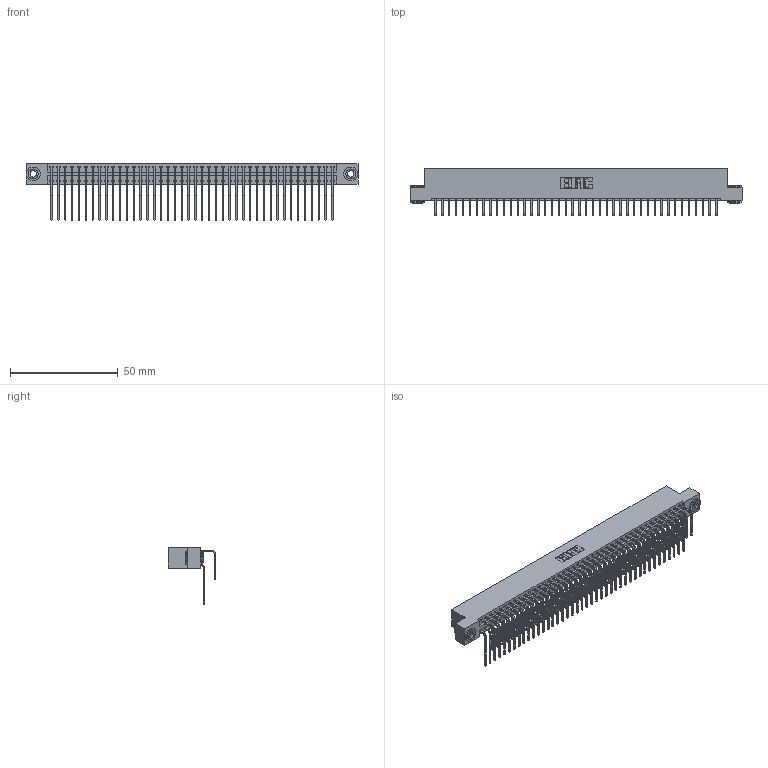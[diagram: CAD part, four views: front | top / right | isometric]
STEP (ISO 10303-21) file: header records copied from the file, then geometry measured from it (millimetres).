
FILE_DESCRIPTION (( 'STEP AP203' ), '1' );
FILE_NAME ('346-084-558-203.STEP', '2022-05-25T20:49:17', ( '' ), ( '' ), 'SwSTEP 2.0', 'SolidWorks 2020', '' );
FILE_SCHEMA (( 'CONFIG_CONTROL_DESIGN' ));
Length unit declared in the file: inch
Products named in the file (5): 346-084-558-203; 345-292-001_558 Tail - 2; 345-250-002_345-250-002-102; 345-292-001_558 559 Tail - 1; 346 Part_Flush Mounting Lugs - 0.156 Dia-TH
Assembly tree (87 placements, depth 2):
  346-084-558-203
    346 Part_Flush Mounting Lugs - 0.156 Dia-TH
    345-292-001_558 559 Tail - 1  x42
    345-292-001_558 Tail - 2  x42
    345-250-002_345-250-002-102  x2
Bounding box: 153.92 x 22.16 x 26.16 mm (x, y, z)
Volume: 15495.4 mm3; surface area: 23872.8 mm2
Topology: 87 solids, 87 shells, 4710 faces, 13965 edges, 9194 vertices
Faces by surface type: plane 3208, cylinder 1494, cone 8
Entity records: 30260 total; most frequent: CARTESIAN_POINT 5020, ORIENTED_EDGE 4894, DIRECTION 4477, EDGE_CURVE 2447, VECTOR 2083, LINE 2083, VERTEX_POINT 1626, AXIS2_PLACEMENT_3D 1197
